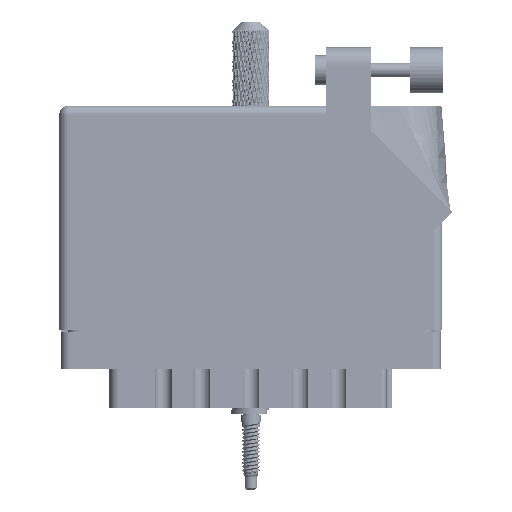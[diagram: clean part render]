
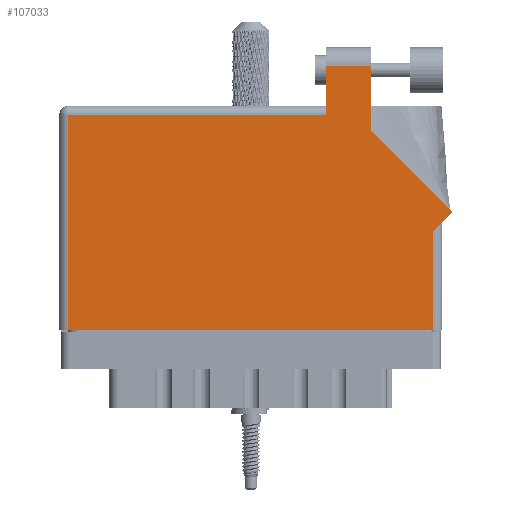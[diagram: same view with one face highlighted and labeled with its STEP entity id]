
A CAD part, front view. The second image highlights one B-rep face of the part: STEP entity #107033.
In plain terms, the highlighted face is planar.
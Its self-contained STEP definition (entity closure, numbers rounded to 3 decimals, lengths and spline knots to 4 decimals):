
#778 = DIRECTION ( 'NONE',  ( -1., 0., 0. ) ) ;
#1075 = ORIENTED_EDGE ( 'NONE', *, *, #44434, .T. ) ;
#1506 = AXIS2_PLACEMENT_3D ( 'NONE', #42827, #15776, #71773 ) ;
#2593 = ORIENTED_EDGE ( 'NONE', *, *, #54798, .T. ) ;
#3062 = VERTEX_POINT ( 'NONE', #102557 ) ;
#4217 = ORIENTED_EDGE ( 'NONE', *, *, #16498, .T. ) ;
#5253 = CARTESIAN_POINT ( 'NONE',  ( 1.819, 1.468, 0. ) ) ;
#6104 = PLANE ( 'NONE',  #1506 ) ;
#6314 = DIRECTION ( 'NONE',  ( 0., -1., 0. ) ) ;
#7192 = VERTEX_POINT ( 'NONE', #18667 ) ;
#10142 = EDGE_CURVE ( 'NONE', #58250, #110332, #116975, .T. ) ;
#11589 = LINE ( 'NONE', #63071, #70512 ) ;
#11740 = EDGE_LOOP ( 'NONE', ( #4217, #62357, #2593, #61770, #22738, #64634, #50326, #1075, #101492 ) ) ;
#11827 = CARTESIAN_POINT ( 'NONE',  ( 2.612, 0.737, 0. ) ) ;
#15776 = DIRECTION ( 'NONE',  ( 0., 0., -1. ) ) ;
#15851 = DIRECTION ( 'NONE',  ( 0., 1., 0. ) ) ;
#16498 = EDGE_CURVE ( 'NONE', #73907, #60871, #97192, .T. ) ;
#17844 = LINE ( 'NONE', #61794, #63953 ) ;
#18460 = LINE ( 'NONE', #85302, #76095 ) ;
#18667 = CARTESIAN_POINT ( 'NONE',  ( 1.819, 1.805, 0. ) ) ;
#20102 = LINE ( 'NONE', #27434, #115086 ) ;
#21315 = LINE ( 'NONE', #11827, #91818 ) ;
#21951 = VECTOR ( 'NONE', #6314, 39.3701 ) ;
#22282 = VECTOR ( 'NONE', #110711, 39.3701 ) ;
#22738 = ORIENTED_EDGE ( 'NONE', *, *, #10142, .T. ) ;
#26566 = DIRECTION ( 'NONE',  ( -1., 0., 0. ) ) ;
#27434 = CARTESIAN_POINT ( 'NONE',  ( 0., 1.468, 0. ) ) ;
#28834 = DIRECTION ( 'NONE',  ( 0., 1., 0. ) ) ;
#29466 = LINE ( 'NONE', #118792, #22282 ) ;
#32238 = EDGE_CURVE ( 'NONE', #51586, #114077, #17844, .T. ) ;
#36411 = CARTESIAN_POINT ( 'NONE',  ( 0.062, 0., 0. ) ) ;
#41471 = CARTESIAN_POINT ( 'NONE',  ( 2.126, 1.3644, 0. ) ) ;
#42827 = CARTESIAN_POINT ( 'NONE',  ( 0., 1.53, 0. ) ) ;
#44434 = EDGE_CURVE ( 'NONE', #114077, #3062, #21315, .T. ) ;
#47571 = CARTESIAN_POINT ( 'NONE',  ( 2.55, 0.675, 0. ) ) ;
#48974 = EDGE_CURVE ( 'NONE', #110332, #51586, #11589, .T. ) ;
#50326 = ORIENTED_EDGE ( 'NONE', *, *, #32238, .T. ) ;
#51586 = VERTEX_POINT ( 'NONE', #102279 ) ;
#51802 = EDGE_CURVE ( 'NONE', #3062, #73907, #18460, .T. ) ;
#54581 = CARTESIAN_POINT ( 'NONE',  ( 0.062, 1.468, 0. ) ) ;
#54798 = EDGE_CURVE ( 'NONE', #7192, #89760, #29466, .T. ) ;
#55420 = CARTESIAN_POINT ( 'NONE',  ( 2.126, 1.805, 0. ) ) ;
#58250 = VERTEX_POINT ( 'NONE', #54581 ) ;
#58581 = LINE ( 'NONE', #82775, #113298 ) ;
#60871 = VERTEX_POINT ( 'NONE', #55420 ) ;
#61770 = ORIENTED_EDGE ( 'NONE', *, *, #95634, .T. ) ;
#61794 = CARTESIAN_POINT ( 'NONE',  ( 2.55, 0.737, 0. ) ) ;
#62357 = ORIENTED_EDGE ( 'NONE', *, *, #103949, .T. ) ;
#63071 = CARTESIAN_POINT ( 'NONE',  ( 0., 0., 0. ) ) ;
#63953 = VECTOR ( 'NONE', #15851, 39.3701 ) ;
#64471 = FACE_OUTER_BOUND ( 'NONE', #11740, .T. ) ;
#64634 = ORIENTED_EDGE ( 'NONE', *, *, #48974, .T. ) ;
#65600 = VECTOR ( 'NONE', #28834, 39.3701 ) ;
#70512 = VECTOR ( 'NONE', #118560, 39.3701 ) ;
#71773 = DIRECTION ( 'NONE',  ( -1., 0., 0. ) ) ;
#73907 = VERTEX_POINT ( 'NONE', #41471 ) ;
#76095 = VECTOR ( 'NONE', #115888, 39.3701 ) ;
#79555 = CARTESIAN_POINT ( 'NONE',  ( 0.062, 0., 0. ) ) ;
#82775 = CARTESIAN_POINT ( 'NONE',  ( 1.819, 1.805, 0. ) ) ;
#85302 = CARTESIAN_POINT ( 'NONE',  ( 2.6827, 0.8077, 0. ) ) ;
#89760 = VERTEX_POINT ( 'NONE', #5253 ) ;
#91818 = VECTOR ( 'NONE', #95516, 39.3701 ) ;
#95516 = DIRECTION ( 'NONE',  ( 0.707, 0.707, 0. ) ) ;
#95634 = EDGE_CURVE ( 'NONE', #89760, #58250, #20102, .T. ) ;
#97192 = LINE ( 'NONE', #107890, #65600 ) ;
#101492 = ORIENTED_EDGE ( 'NONE', *, *, #51802, .T. ) ;
#102279 = CARTESIAN_POINT ( 'NONE',  ( 2.55, 0., 0. ) ) ;
#102557 = CARTESIAN_POINT ( 'NONE',  ( 2.6827, 0.8077, 0. ) ) ;
#103949 = EDGE_CURVE ( 'NONE', #60871, #7192, #58581, .T. ) ;
#107033 = ADVANCED_FACE ( 'NONE', ( #64471 ), #6104, .F. ) ;
#107890 = CARTESIAN_POINT ( 'NONE',  ( 2.126, 1.3644, 0. ) ) ;
#110332 = VERTEX_POINT ( 'NONE', #36411 ) ;
#110711 = DIRECTION ( 'NONE',  ( 0., -1., 0. ) ) ;
#113298 = VECTOR ( 'NONE', #26566, 39.3701 ) ;
#114077 = VERTEX_POINT ( 'NONE', #47571 ) ;
#115086 = VECTOR ( 'NONE', #778, 39.3701 ) ;
#115888 = DIRECTION ( 'NONE',  ( -0.707, 0.707, 0. ) ) ;
#116975 = LINE ( 'NONE', #79555, #21951 ) ;
#118560 = DIRECTION ( 'NONE',  ( 1., 0., 0. ) ) ;
#118792 = CARTESIAN_POINT ( 'NONE',  ( 1.819, 1.53, 0. ) ) ;
